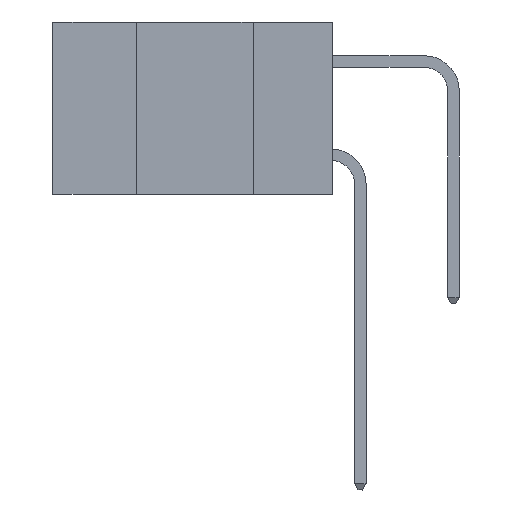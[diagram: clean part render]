
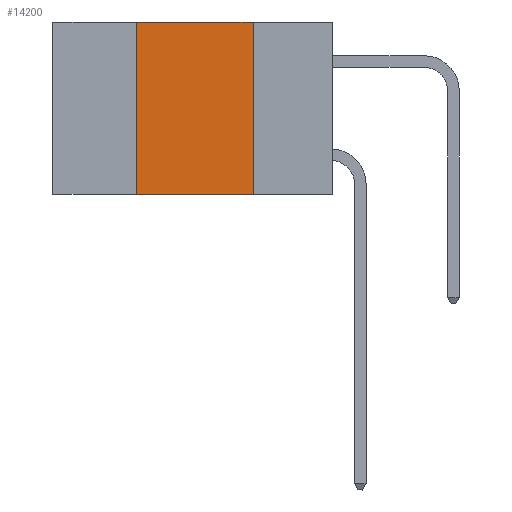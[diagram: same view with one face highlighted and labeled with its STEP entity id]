
A CAD part, left-side view. The second image highlights one B-rep face of the part: STEP entity #14200.
In plain terms, the highlighted planar face has unit normal (-1, 0, 0).
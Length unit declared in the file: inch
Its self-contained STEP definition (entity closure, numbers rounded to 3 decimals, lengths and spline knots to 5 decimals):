
#467 = CARTESIAN_POINT ( 'NONE',  ( 0., 0.6, 0. ) ) ;
#1694 = ORIENTED_EDGE ( 'NONE', *, *, #9073, .F. ) ;
#2143 = VECTOR ( 'NONE', #22071, 39.37008 ) ;
#3661 = CARTESIAN_POINT ( 'NONE',  ( 0., 0.17, 0. ) ) ;
#3691 = VERTEX_POINT ( 'NONE', #26275 ) ;
#4603 = ORIENTED_EDGE ( 'NONE', *, *, #18148, .T. ) ;
#4640 = ORIENTED_EDGE ( 'NONE', *, *, #23047, .F. ) ;
#4882 = EDGE_CURVE ( 'NONE', #3691, #24061, #21133, .T. ) ;
#6567 = DIRECTION ( 'NONE',  ( 0., -1., 0. ) ) ;
#7796 = VERTEX_POINT ( 'NONE', #3661 ) ;
#8507 = CARTESIAN_POINT ( 'NONE',  ( 0., 0.6, 0. ) ) ;
#8758 = VECTOR ( 'NONE', #11283, 39.37008 ) ;
#9073 = EDGE_CURVE ( 'NONE', #7796, #13753, #17654, .T. ) ;
#9094 = CARTESIAN_POINT ( 'NONE',  ( 0., 0.6, -0.37 ) ) ;
#9651 = LINE ( 'NONE', #8507, #14614 ) ;
#11283 = DIRECTION ( 'NONE',  ( 0., 0., -1. ) ) ;
#12310 = AXIS2_PLACEMENT_3D ( 'NONE', #467, #19401, #17620 ) ;
#13753 = VERTEX_POINT ( 'NONE', #23794 ) ;
#14200 = ADVANCED_FACE ( 'NONE', ( #20004 ), #15527, .F. ) ;
#14498 = VECTOR ( 'NONE', #14582, 39.37008 ) ;
#14582 = DIRECTION ( 'NONE',  ( 0., 0., 1. ) ) ;
#14614 = VECTOR ( 'NONE', #6567, 39.37008 ) ;
#15527 = PLANE ( 'NONE',  #12310 ) ;
#17620 = DIRECTION ( 'NONE',  ( 0., 0., -1. ) ) ;
#17654 = LINE ( 'NONE', #19772, #8758 ) ;
#18148 = EDGE_CURVE ( 'NONE', #3691, #13753, #22242, .T. ) ;
#19401 = DIRECTION ( 'NONE',  ( 1., 0., 0. ) ) ;
#19772 = CARTESIAN_POINT ( 'NONE',  ( 0., 0.17, 0. ) ) ;
#20004 = FACE_OUTER_BOUND ( 'NONE', #20813, .T. ) ;
#20813 = EDGE_LOOP ( 'NONE', ( #1694, #4640, #22253, #4603 ) ) ;
#21133 = LINE ( 'NONE', #25068, #14498 ) ;
#22071 = DIRECTION ( 'NONE',  ( 0., -1., 0. ) ) ;
#22242 = LINE ( 'NONE', #9094, #2143 ) ;
#22253 = ORIENTED_EDGE ( 'NONE', *, *, #4882, .F. ) ;
#23047 = EDGE_CURVE ( 'NONE', #24061, #7796, #9651, .T. ) ;
#23794 = CARTESIAN_POINT ( 'NONE',  ( 0., 0.17, -0.37 ) ) ;
#24061 = VERTEX_POINT ( 'NONE', #25542 ) ;
#25068 = CARTESIAN_POINT ( 'NONE',  ( 0., 0.42, 0. ) ) ;
#25542 = CARTESIAN_POINT ( 'NONE',  ( 0., 0.42, 0. ) ) ;
#26275 = CARTESIAN_POINT ( 'NONE',  ( 0., 0.42, -0.37 ) ) ;
